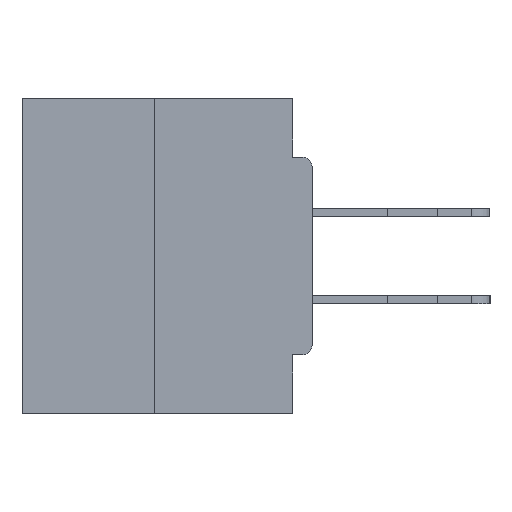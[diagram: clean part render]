
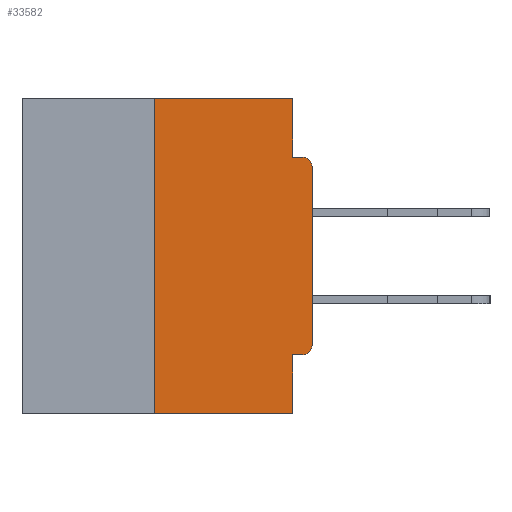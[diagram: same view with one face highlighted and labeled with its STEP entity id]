
A CAD part, left-side view. The second image highlights one B-rep face of the part: STEP entity #33582.
In plain terms, the highlighted planar face has unit normal (-1, 0, 0).
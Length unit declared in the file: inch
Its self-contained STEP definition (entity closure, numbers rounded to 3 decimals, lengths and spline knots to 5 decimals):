
#305 = ORIENTED_EDGE ( 'NONE', *, *, #11485, .F. ) ;
#320 = EDGE_CURVE ( 'NONE', #5353, #6400, #12555, .T. ) ;
#526 = EDGE_CURVE ( 'NONE', #6518, #6850, #6772, .T. ) ;
#2446 = DIRECTION ( 'NONE',  ( 0., 0., -1. ) ) ;
#4145 = PLANE ( 'NONE',  #29350 ) ;
#4695 = CARTESIAN_POINT ( 'NONE',  ( 0., 0.015, -0.0935 ) ) ;
#5353 = VERTEX_POINT ( 'NONE', #7888 ) ;
#5441 = VECTOR ( 'NONE', #7181, 39.37008 ) ;
#5517 = VERTEX_POINT ( 'NONE', #19317 ) ;
#5519 = CARTESIAN_POINT ( 'NONE',  ( 0., 0.46, 0. ) ) ;
#5860 = LINE ( 'NONE', #29166, #27303 ) ;
#6199 = VECTOR ( 'NONE', #12712, 39.37008 ) ;
#6255 = LINE ( 'NONE', #12628, #5441 ) ;
#6400 = VERTEX_POINT ( 'NONE', #4695 ) ;
#6518 = VERTEX_POINT ( 'NONE', #31434 ) ;
#6772 = LINE ( 'NONE', #21520, #13816 ) ;
#6850 = VERTEX_POINT ( 'NONE', #18317 ) ;
#7001 = CARTESIAN_POINT ( 'NONE',  ( 0., 0.015, -0.1085 ) ) ;
#7117 = CARTESIAN_POINT ( 'NONE',  ( 0., 0.031, 0. ) ) ;
#7181 = DIRECTION ( 'NONE',  ( 0., 0., 1. ) ) ;
#7888 = CARTESIAN_POINT ( 'NONE',  ( 0., 0., -0.1085 ) ) ;
#7981 = VECTOR ( 'NONE', #10879, 39.37008 ) ;
#8469 = VERTEX_POINT ( 'NONE', #11349 ) ;
#9129 = DIRECTION ( 'NONE',  ( 0., 0., -1. ) ) ;
#9318 = ORIENTED_EDGE ( 'NONE', *, *, #526, .F. ) ;
#9662 = DIRECTION ( 'NONE',  ( 0., 0., -1. ) ) ;
#9791 = EDGE_CURVE ( 'NONE', #5517, #6850, #15773, .T. ) ;
#10185 = VERTEX_POINT ( 'NONE', #7117 ) ;
#10879 = DIRECTION ( 'NONE',  ( 0., 0., 1. ) ) ;
#11349 = CARTESIAN_POINT ( 'NONE',  ( 0., 0., -0.3915 ) ) ;
#11485 = EDGE_CURVE ( 'NONE', #15933, #10185, #16538, .T. ) ;
#12555 = CIRCLE ( 'NONE', #33510, 0.015 ) ;
#12628 = CARTESIAN_POINT ( 'NONE',  ( 0., 0., 0. ) ) ;
#12639 = EDGE_LOOP ( 'NONE', ( #305, #21312, #14556, #9318, #34180, #21444, #32627, #24669, #28628, #31148 ) ) ;
#12712 = DIRECTION ( 'NONE',  ( 0., -1., 0. ) ) ;
#13816 = VECTOR ( 'NONE', #26826, 39.37008 ) ;
#13957 = CARTESIAN_POINT ( 'NONE',  ( 0., 0.25, 0. ) ) ;
#14556 = ORIENTED_EDGE ( 'NONE', *, *, #9791, .T. ) ;
#15012 = EDGE_CURVE ( 'NONE', #10185, #18979, #26740, .T. ) ;
#15773 = LINE ( 'NONE', #31750, #30587 ) ;
#15809 = CARTESIAN_POINT ( 'NONE',  ( 0., 0.25, 0. ) ) ;
#15919 = CIRCLE ( 'NONE', #16527, 0.015 ) ;
#15930 = CARTESIAN_POINT ( 'NONE',  ( 0., 0.031, -0.0935 ) ) ;
#15933 = VERTEX_POINT ( 'NONE', #13957 ) ;
#16272 = DIRECTION ( 'NONE',  ( 0., -1., 0. ) ) ;
#16527 = AXIS2_PLACEMENT_3D ( 'NONE', #26345, #23457, #26114 ) ;
#16538 = LINE ( 'NONE', #5519, #32197 ) ;
#18317 = CARTESIAN_POINT ( 'NONE',  ( 0., 0.031, -0.5 ) ) ;
#18678 = DIRECTION ( 'NONE',  ( 0., 1., 0. ) ) ;
#18951 = VERTEX_POINT ( 'NONE', #24213 ) ;
#18979 = VERTEX_POINT ( 'NONE', #15930 ) ;
#19317 = CARTESIAN_POINT ( 'NONE',  ( 0., 0.25, -0.5 ) ) ;
#19505 = DIRECTION ( 'NONE',  ( 1., 0., 0. ) ) ;
#19743 = VECTOR ( 'NONE', #2446, 39.37008 ) ;
#20318 = EDGE_CURVE ( 'NONE', #5517, #15933, #26978, .T. ) ;
#20521 = DIRECTION ( 'NONE',  ( -1., 0., 0. ) ) ;
#21312 = ORIENTED_EDGE ( 'NONE', *, *, #20318, .F. ) ;
#21377 = EDGE_CURVE ( 'NONE', #18951, #6518, #5860, .T. ) ;
#21444 = ORIENTED_EDGE ( 'NONE', *, *, #26827, .T. ) ;
#21520 = CARTESIAN_POINT ( 'NONE',  ( 0., 0.031, -0.5 ) ) ;
#23427 = CARTESIAN_POINT ( 'NONE',  ( 0., 0.031, 0. ) ) ;
#23457 = DIRECTION ( 'NONE',  ( -1., 0., 0. ) ) ;
#23583 = DIRECTION ( 'NONE',  ( 0., -1., 0. ) ) ;
#24213 = CARTESIAN_POINT ( 'NONE',  ( 0., 0.015, -0.4065 ) ) ;
#24669 = ORIENTED_EDGE ( 'NONE', *, *, #320, .T. ) ;
#25487 = FACE_OUTER_BOUND ( 'NONE', #12639, .T. ) ;
#26114 = DIRECTION ( 'NONE',  ( 0., 0., -1. ) ) ;
#26345 = CARTESIAN_POINT ( 'NONE',  ( 0., 0.015, -0.3915 ) ) ;
#26740 = LINE ( 'NONE', #23427, #19743 ) ;
#26826 = DIRECTION ( 'NONE',  ( 0., 0., -1. ) ) ;
#26827 = EDGE_CURVE ( 'NONE', #18951, #8469, #15919, .T. ) ;
#26978 = LINE ( 'NONE', #15809, #7981 ) ;
#27303 = VECTOR ( 'NONE', #18678, 39.37008 ) ;
#28628 = ORIENTED_EDGE ( 'NONE', *, *, #31319, .F. ) ;
#29166 = CARTESIAN_POINT ( 'NONE',  ( 0., 0., -0.4065 ) ) ;
#29350 = AXIS2_PLACEMENT_3D ( 'NONE', #30541, #19505, #9129 ) ;
#30111 = LINE ( 'NONE', #31016, #6199 ) ;
#30525 = EDGE_CURVE ( 'NONE', #8469, #5353, #6255, .T. ) ;
#30541 = CARTESIAN_POINT ( 'NONE',  ( 0., 0.46, 0. ) ) ;
#30587 = VECTOR ( 'NONE', #23583, 39.37008 ) ;
#31016 = CARTESIAN_POINT ( 'NONE',  ( 0., 0., -0.0935 ) ) ;
#31148 = ORIENTED_EDGE ( 'NONE', *, *, #15012, .F. ) ;
#31319 = EDGE_CURVE ( 'NONE', #18979, #6400, #30111, .T. ) ;
#31434 = CARTESIAN_POINT ( 'NONE',  ( 0., 0.031, -0.4065 ) ) ;
#31750 = CARTESIAN_POINT ( 'NONE',  ( 0., 0.46, -0.5 ) ) ;
#32197 = VECTOR ( 'NONE', #16272, 39.37008 ) ;
#32627 = ORIENTED_EDGE ( 'NONE', *, *, #30525, .T. ) ;
#33510 = AXIS2_PLACEMENT_3D ( 'NONE', #7001, #20521, #9662 ) ;
#33582 = ADVANCED_FACE ( 'NONE', ( #25487 ), #4145, .F. ) ;
#34180 = ORIENTED_EDGE ( 'NONE', *, *, #21377, .F. ) ;
